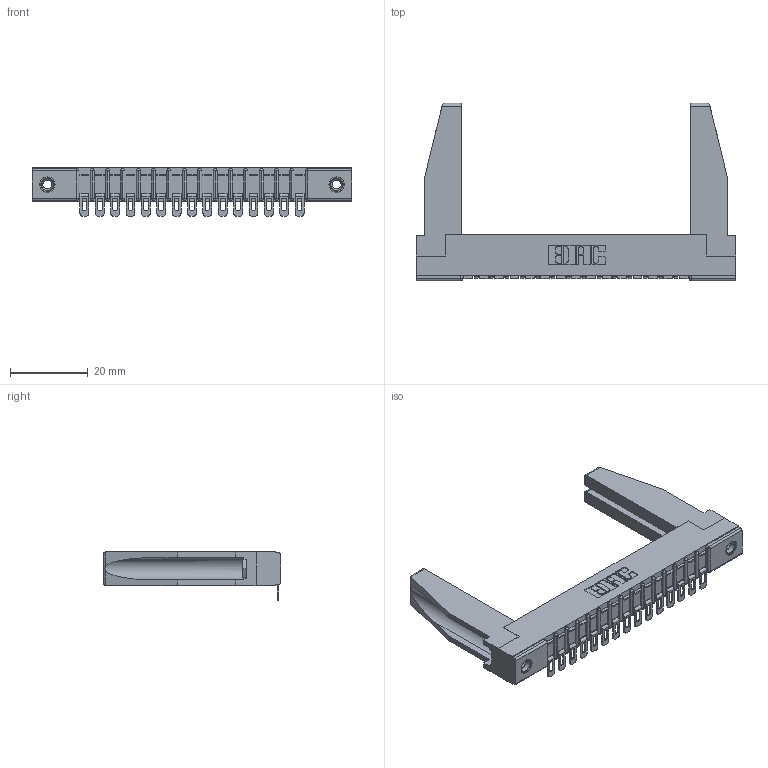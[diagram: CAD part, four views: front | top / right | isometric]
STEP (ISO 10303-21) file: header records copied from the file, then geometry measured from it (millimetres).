
FILE_DESCRIPTION (( 'STEP AP203' ), '1' );
FILE_NAME ('357-015-454-178.STEP', '2020-09-30T18:17:32', ( '' ), ( '' ), 'SwSTEP 2.0', 'SolidWorks 2020', '' );
FILE_SCHEMA (( 'CONFIG_CONTROL_DESIGN' ));
Length unit declared in the file: inch
Products named in the file (5): 307-290-002_554; 357-015-454-178; 307-220-078; 345-250-001_345-250-001-102; 307 Part_.156 Dia Mounting Holes
Assembly tree (20 placements, depth 2):
  357-015-454-178
    307 Part_.156 Dia Mounting Holes
    307-290-002_554  x15
    307-220-078  x2
    345-250-001_345-250-001-102  x2
Bounding box: 82.45 x 45.72 x 12.52 mm (x, y, z)
Volume: 9438.2 mm3; surface area: 13396.5 mm2
Topology: 20 solids, 20 shells, 1479 faces, 4448 edges, 2912 vertices
Faces by surface type: plane 844, cylinder 587, sphere 32, cone 12, torus 4
Entity records: 19592 total; most frequent: CARTESIAN_POINT 3300, ORIENTED_EDGE 3246, DIRECTION 3181, EDGE_CURVE 1623, LINE 1227, VECTOR 1227, VERTEX_POINT 1054, AXIS2_PLACEMENT_3D 977
